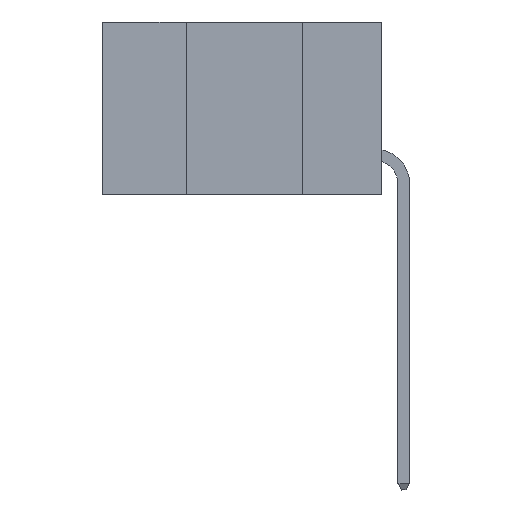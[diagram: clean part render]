
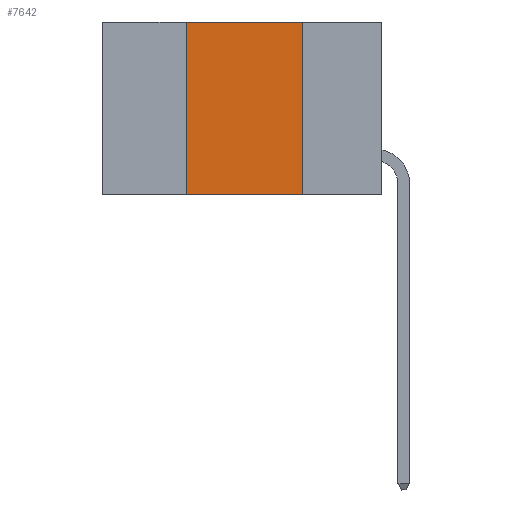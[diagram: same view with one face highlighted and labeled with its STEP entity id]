
A CAD part, left-side view. The second image highlights one B-rep face of the part: STEP entity #7642.
In plain terms, the highlighted planar face has unit normal (-1, 0, 0).
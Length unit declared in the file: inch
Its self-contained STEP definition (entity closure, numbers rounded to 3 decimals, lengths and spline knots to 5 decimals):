
#2092 = EDGE_CURVE ( 'NONE', #16786, #10644, #6184, .T. ) ;
#2790 = LINE ( 'NONE', #12934, #12256 ) ;
#3146 = CARTESIAN_POINT ( 'NONE',  ( 0., 0.42, 0. ) ) ;
#3608 = LINE ( 'NONE', #17843, #9829 ) ;
#3721 = AXIS2_PLACEMENT_3D ( 'NONE', #4026, #9518, #13856 ) ;
#3767 = PLANE ( 'NONE',  #3721 ) ;
#3928 = DIRECTION ( 'NONE',  ( 0., 0., -1. ) ) ;
#4026 = CARTESIAN_POINT ( 'NONE',  ( 0., 0.6, 0. ) ) ;
#6184 = LINE ( 'NONE', #13880, #12306 ) ;
#6634 = CARTESIAN_POINT ( 'NONE',  ( 0., 0.17, 0. ) ) ;
#7642 = ADVANCED_FACE ( 'NONE', ( #14188 ), #3767, .F. ) ;
#8094 = CARTESIAN_POINT ( 'NONE',  ( 0., 0.42, -0.37 ) ) ;
#8853 = ORIENTED_EDGE ( 'NONE', *, *, #2092, .F. ) ;
#8987 = DIRECTION ( 'NONE',  ( 0., 0., 1. ) ) ;
#9367 = DIRECTION ( 'NONE',  ( 0., -1., 0. ) ) ;
#9518 = DIRECTION ( 'NONE',  ( 1., 0., 0. ) ) ;
#9829 = VECTOR ( 'NONE', #9367, 39.37008 ) ;
#10644 = VERTEX_POINT ( 'NONE', #15464 ) ;
#11175 = ORIENTED_EDGE ( 'NONE', *, *, #15234, .F. ) ;
#11528 = ORIENTED_EDGE ( 'NONE', *, *, #12354, .F. ) ;
#11600 = EDGE_CURVE ( 'NONE', #11986, #10644, #15789, .T. ) ;
#11986 = VERTEX_POINT ( 'NONE', #8094 ) ;
#12041 = VECTOR ( 'NONE', #15078, 39.37008 ) ;
#12256 = VECTOR ( 'NONE', #8987, 39.37008 ) ;
#12306 = VECTOR ( 'NONE', #3928, 39.37008 ) ;
#12354 = EDGE_CURVE ( 'NONE', #17575, #16786, #3608, .T. ) ;
#12934 = CARTESIAN_POINT ( 'NONE',  ( 0., 0.42, 0. ) ) ;
#13856 = DIRECTION ( 'NONE',  ( 0., 0., -1. ) ) ;
#13880 = CARTESIAN_POINT ( 'NONE',  ( 0., 0.17, 0. ) ) ;
#13972 = ORIENTED_EDGE ( 'NONE', *, *, #11600, .T. ) ;
#14188 = FACE_OUTER_BOUND ( 'NONE', #16904, .T. ) ;
#15078 = DIRECTION ( 'NONE',  ( 0., -1., 0. ) ) ;
#15234 = EDGE_CURVE ( 'NONE', #11986, #17575, #2790, .T. ) ;
#15464 = CARTESIAN_POINT ( 'NONE',  ( 0., 0.17, -0.37 ) ) ;
#15789 = LINE ( 'NONE', #17908, #12041 ) ;
#16786 = VERTEX_POINT ( 'NONE', #6634 ) ;
#16904 = EDGE_LOOP ( 'NONE', ( #8853, #11528, #11175, #13972 ) ) ;
#17575 = VERTEX_POINT ( 'NONE', #3146 ) ;
#17843 = CARTESIAN_POINT ( 'NONE',  ( 0., 0.6, 0. ) ) ;
#17908 = CARTESIAN_POINT ( 'NONE',  ( 0., 0.6, -0.37 ) ) ;
